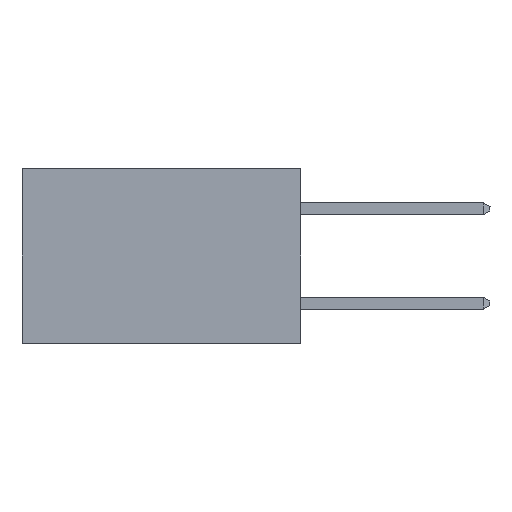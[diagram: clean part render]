
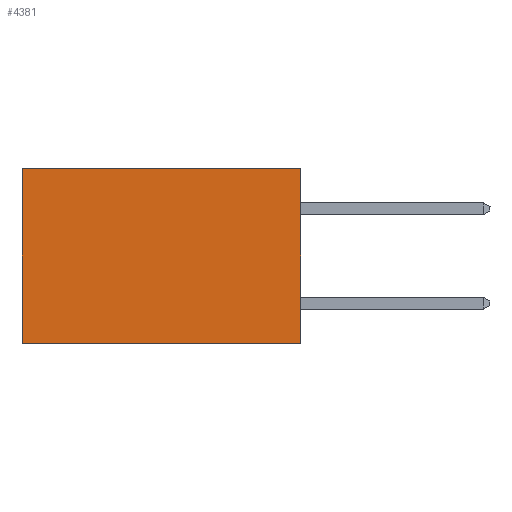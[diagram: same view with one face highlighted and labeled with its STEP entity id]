
A CAD part, left-side view. The second image highlights one B-rep face of the part: STEP entity #4381.
In plain terms, the highlighted planar face has unit normal (-1, 0, 0).
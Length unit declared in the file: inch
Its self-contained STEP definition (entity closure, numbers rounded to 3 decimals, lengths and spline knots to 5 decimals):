
#625 = DIRECTION ( 'NONE',  ( 0., 1., 0. ) ) ;
#707 = VECTOR ( 'NONE', #1114, 39.37008 ) ;
#812 = CARTESIAN_POINT ( 'NONE',  ( 0.277, 0., -0.37 ) ) ;
#1023 = CARTESIAN_POINT ( 'NONE',  ( 0.277, 0., 0. ) ) ;
#1114 = DIRECTION ( 'NONE',  ( 0., 1., 0. ) ) ;
#1787 = CARTESIAN_POINT ( 'NONE',  ( 0.277, 0.59, -0.37 ) ) ;
#1945 = LINE ( 'NONE', #6364, #4680 ) ;
#2299 = VECTOR ( 'NONE', #625, 39.37008 ) ;
#2369 = FACE_OUTER_BOUND ( 'NONE', #8658, .T. ) ;
#2610 = VERTEX_POINT ( 'NONE', #1787 ) ;
#3251 = EDGE_CURVE ( 'NONE', #7483, #11639, #8716, .T. ) ;
#3276 = LINE ( 'NONE', #9822, #11110 ) ;
#3759 = CARTESIAN_POINT ( 'NONE',  ( 0.277, 0., 0. ) ) ;
#4381 = ADVANCED_FACE ( 'NONE', ( #2369 ), #12433, .F. ) ;
#4680 = VECTOR ( 'NONE', #7432, 39.37008 ) ;
#5034 = LINE ( 'NONE', #812, #2299 ) ;
#6364 = CARTESIAN_POINT ( 'NONE',  ( 0.277, 0.59, -0.37 ) ) ;
#6496 = CARTESIAN_POINT ( 'NONE',  ( 0.277, 0., -0.37 ) ) ;
#7432 = DIRECTION ( 'NONE',  ( 0., 0., -1. ) ) ;
#7483 = VERTEX_POINT ( 'NONE', #1023 ) ;
#7517 = EDGE_CURVE ( 'NONE', #10038, #2610, #5034, .T. ) ;
#8658 = EDGE_LOOP ( 'NONE', ( #9104, #9209, #8978, #8965 ) ) ;
#8716 = LINE ( 'NONE', #3759, #707 ) ;
#8965 = ORIENTED_EDGE ( 'NONE', *, *, #3251, .T. ) ;
#8978 = ORIENTED_EDGE ( 'NONE', *, *, #9168, .F. ) ;
#9104 = ORIENTED_EDGE ( 'NONE', *, *, #9888, .T. ) ;
#9168 = EDGE_CURVE ( 'NONE', #7483, #10038, #3276, .T. ) ;
#9209 = ORIENTED_EDGE ( 'NONE', *, *, #7517, .F. ) ;
#9822 = CARTESIAN_POINT ( 'NONE',  ( 0.277, 0., -0.37 ) ) ;
#9888 = EDGE_CURVE ( 'NONE', #11639, #2610, #1945, .T. ) ;
#10038 = VERTEX_POINT ( 'NONE', #6496 ) ;
#10830 = DIRECTION ( 'NONE',  ( 0., 0., -1. ) ) ;
#10961 = AXIS2_PLACEMENT_3D ( 'NONE', #11776, #11683, #11601 ) ;
#11110 = VECTOR ( 'NONE', #10830, 39.37008 ) ;
#11601 = DIRECTION ( 'NONE',  ( 0., 0., -1. ) ) ;
#11639 = VERTEX_POINT ( 'NONE', #12409 ) ;
#11683 = DIRECTION ( 'NONE',  ( 1., 0., 0. ) ) ;
#11776 = CARTESIAN_POINT ( 'NONE',  ( 0.277, 0., -0.37 ) ) ;
#12409 = CARTESIAN_POINT ( 'NONE',  ( 0.277, 0.59, 0. ) ) ;
#12433 = PLANE ( 'NONE',  #10961 ) ;
